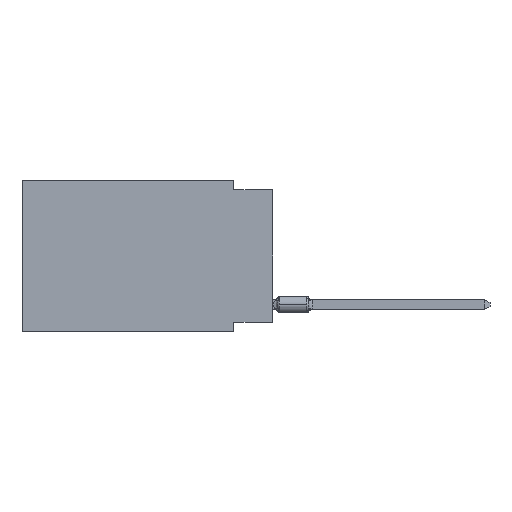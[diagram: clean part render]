
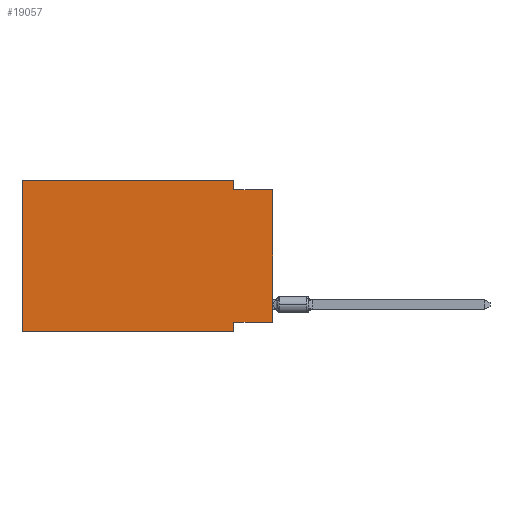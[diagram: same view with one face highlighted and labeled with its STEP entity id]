
A CAD part, left-side view. The second image highlights one B-rep face of the part: STEP entity #19057.
In plain terms, the highlighted planar face has unit normal (-1, 0, 0).
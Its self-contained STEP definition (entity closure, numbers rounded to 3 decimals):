
#77 = CARTESIAN_POINT ( 'NONE',  ( 0., 16.383, 0. ) ) ;
#136 = LINE ( 'NONE', #5096, #19911 ) ;
#178 = PLANE ( 'NONE',  #4351 ) ;
#219 = DIRECTION ( 'NONE',  ( 0., -1., 0. ) ) ;
#351 = CARTESIAN_POINT ( 'NONE',  ( 0., 2.54, 0. ) ) ;
#370 = CARTESIAN_POINT ( 'NONE',  ( 0., 2.54, -9.906 ) ) ;
#1481 = VECTOR ( 'NONE', #219, 1000. ) ;
#1796 = LINE ( 'NONE', #12760, #1481 ) ;
#2210 = LINE ( 'NONE', #13381, #16753 ) ;
#2353 = DIRECTION ( 'NONE',  ( 0., 0., -1. ) ) ;
#2507 = DIRECTION ( 'NONE',  ( 0., -1., 0. ) ) ;
#3294 = EDGE_LOOP ( 'NONE', ( #3913, #17922, #15539, #16948, #8945, #18914, #6197, #11858 ) ) ;
#3522 = DIRECTION ( 'NONE',  ( 0., 0., -1. ) ) ;
#3712 = VERTEX_POINT ( 'NONE', #4319 ) ;
#3812 = CARTESIAN_POINT ( 'NONE',  ( 0., 0., -9.271 ) ) ;
#3913 = ORIENTED_EDGE ( 'NONE', *, *, #13043, .T. ) ;
#4319 = CARTESIAN_POINT ( 'NONE',  ( 0., 16.383, -9.906 ) ) ;
#4351 = AXIS2_PLACEMENT_3D ( 'NONE', #77, #11937, #2353 ) ;
#4633 = VERTEX_POINT ( 'NONE', #7243 ) ;
#4683 = CARTESIAN_POINT ( 'NONE',  ( 0., 2.54, -9.271 ) ) ;
#4731 = VERTEX_POINT ( 'NONE', #4683 ) ;
#4792 = EDGE_CURVE ( 'NONE', #8056, #4731, #19161, .T. ) ;
#4930 = FACE_OUTER_BOUND ( 'NONE', #3294, .T. ) ;
#5010 = CARTESIAN_POINT ( 'NONE',  ( 0., 0., -0.635 ) ) ;
#5096 = CARTESIAN_POINT ( 'NONE',  ( 0., 16.383, 0. ) ) ;
#6020 = EDGE_CURVE ( 'NONE', #16587, #17694, #18090, .T. ) ;
#6197 = ORIENTED_EDGE ( 'NONE', *, *, #15104, .F. ) ;
#7243 = CARTESIAN_POINT ( 'NONE',  ( 0., 16.383, 0. ) ) ;
#7359 = CARTESIAN_POINT ( 'NONE',  ( 0., 2.54, -0.635 ) ) ;
#7610 = VERTEX_POINT ( 'NONE', #5010 ) ;
#8056 = VERTEX_POINT ( 'NONE', #3812 ) ;
#8945 = ORIENTED_EDGE ( 'NONE', *, *, #14336, .F. ) ;
#9196 = DIRECTION ( 'NONE',  ( 0., 0., 1. ) ) ;
#9661 = EDGE_CURVE ( 'NONE', #3712, #18411, #18674, .T. ) ;
#9700 = CARTESIAN_POINT ( 'NONE',  ( 0., 0., -9.271 ) ) ;
#10336 = VECTOR ( 'NONE', #2507, 1000. ) ;
#10799 = CARTESIAN_POINT ( 'NONE',  ( 0., 0., 0. ) ) ;
#11117 = VECTOR ( 'NONE', #16613, 1000. ) ;
#11408 = EDGE_CURVE ( 'NONE', #17694, #7610, #1796, .T. ) ;
#11578 = EDGE_CURVE ( 'NONE', #4633, #16587, #2210, .T. ) ;
#11858 = ORIENTED_EDGE ( 'NONE', *, *, #4792, .F. ) ;
#11937 = DIRECTION ( 'NONE',  ( 1., 0., 0. ) ) ;
#12760 = CARTESIAN_POINT ( 'NONE',  ( 0., 0., -0.635 ) ) ;
#12851 = VECTOR ( 'NONE', #9196, 1000. ) ;
#13043 = EDGE_CURVE ( 'NONE', #8056, #7610, #19079, .T. ) ;
#13273 = DIRECTION ( 'NONE',  ( 0., -1., 0. ) ) ;
#13381 = CARTESIAN_POINT ( 'NONE',  ( 0., 16.383, 0. ) ) ;
#13701 = CARTESIAN_POINT ( 'NONE',  ( 0., 2.54, -9.906 ) ) ;
#14336 = EDGE_CURVE ( 'NONE', #3712, #4633, #136, .T. ) ;
#15104 = EDGE_CURVE ( 'NONE', #4731, #18411, #16300, .T. ) ;
#15539 = ORIENTED_EDGE ( 'NONE', *, *, #6020, .F. ) ;
#16172 = DIRECTION ( 'NONE',  ( 0., 0., 1. ) ) ;
#16300 = LINE ( 'NONE', #370, #11117 ) ;
#16587 = VERTEX_POINT ( 'NONE', #20879 ) ;
#16613 = DIRECTION ( 'NONE',  ( 0., 0., -1. ) ) ;
#16753 = VECTOR ( 'NONE', #13273, 1000. ) ;
#16948 = ORIENTED_EDGE ( 'NONE', *, *, #11578, .F. ) ;
#17076 = CARTESIAN_POINT ( 'NONE',  ( 0., 16.383, -9.906 ) ) ;
#17694 = VERTEX_POINT ( 'NONE', #7359 ) ;
#17922 = ORIENTED_EDGE ( 'NONE', *, *, #11408, .F. ) ;
#18090 = LINE ( 'NONE', #351, #19116 ) ;
#18411 = VERTEX_POINT ( 'NONE', #13701 ) ;
#18674 = LINE ( 'NONE', #17076, #10336 ) ;
#18914 = ORIENTED_EDGE ( 'NONE', *, *, #9661, .T. ) ;
#19057 = ADVANCED_FACE ( 'NONE', ( #4930 ), #178, .F. ) ;
#19079 = LINE ( 'NONE', #10799, #12851 ) ;
#19116 = VECTOR ( 'NONE', #3522, 1000. ) ;
#19161 = LINE ( 'NONE', #9700, #19314 ) ;
#19266 = DIRECTION ( 'NONE',  ( 0., 1., 0. ) ) ;
#19314 = VECTOR ( 'NONE', #19266, 1000. ) ;
#19911 = VECTOR ( 'NONE', #16172, 1000. ) ;
#20879 = CARTESIAN_POINT ( 'NONE',  ( 0., 2.54, 0. ) ) ;
